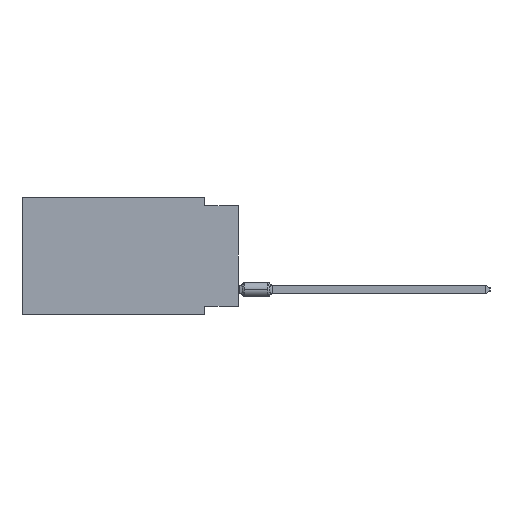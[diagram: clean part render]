
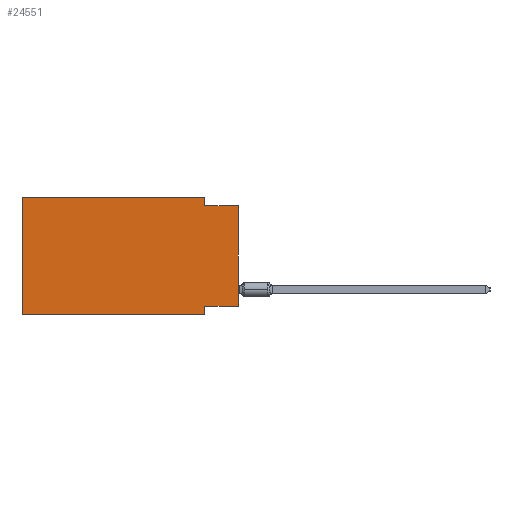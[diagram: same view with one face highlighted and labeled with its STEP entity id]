
A CAD part, left-side view. The second image highlights one B-rep face of the part: STEP entity #24551.
In plain terms, the highlighted planar face has unit normal (-1, 0, 0).
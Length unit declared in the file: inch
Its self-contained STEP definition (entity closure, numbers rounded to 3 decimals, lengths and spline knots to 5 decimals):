
#3722 = CARTESIAN_POINT ( 'NONE',  ( 0., 0.1, -0.35 ) ) ;
#4383 = EDGE_CURVE ( 'NONE', #33869, #52379, #29359, .T. ) ;
#4800 = PLANE ( 'NONE',  #45881 ) ;
#4854 = VECTOR ( 'NONE', #38782, 39.37008 ) ;
#5551 = CARTESIAN_POINT ( 'NONE',  ( 0., 0.645, -0.35 ) ) ;
#7350 = VERTEX_POINT ( 'NONE', #24100 ) ;
#8045 = CARTESIAN_POINT ( 'NONE',  ( 0., 0.645, 0. ) ) ;
#9437 = ORIENTED_EDGE ( 'NONE', *, *, #50084, .F. ) ;
#10578 = ORIENTED_EDGE ( 'NONE', *, *, #64224, .T. ) ;
#11605 = EDGE_CURVE ( 'NONE', #21707, #7350, #18316, .T. ) ;
#14691 = CARTESIAN_POINT ( 'NONE',  ( 0., 0.1, -0.025 ) ) ;
#14820 = DIRECTION ( 'NONE',  ( 0., 0., -1. ) ) ;
#15753 = DIRECTION ( 'NONE',  ( 1., 0., 0. ) ) ;
#16477 = DIRECTION ( 'NONE',  ( 0., 0., -1. ) ) ;
#18316 = LINE ( 'NONE', #50862, #23615 ) ;
#18768 = LINE ( 'NONE', #24285, #55905 ) ;
#21707 = VERTEX_POINT ( 'NONE', #14691 ) ;
#23089 = EDGE_CURVE ( 'NONE', #51325, #28256, #49789, .T. ) ;
#23615 = VECTOR ( 'NONE', #57078, 39.37008 ) ;
#23792 = LINE ( 'NONE', #8045, #57624 ) ;
#23897 = CARTESIAN_POINT ( 'NONE',  ( 0., 0., -0.325 ) ) ;
#24100 = CARTESIAN_POINT ( 'NONE',  ( 0., 0., -0.025 ) ) ;
#24285 = CARTESIAN_POINT ( 'NONE',  ( 0., 0., 0. ) ) ;
#24551 = ADVANCED_FACE ( 'NONE', ( #66188 ), #4800, .F. ) ;
#25277 = EDGE_CURVE ( 'NONE', #49358, #38225, #23792, .T. ) ;
#25859 = EDGE_CURVE ( 'NONE', #51325, #49358, #39706, .T. ) ;
#26925 = ORIENTED_EDGE ( 'NONE', *, *, #23089, .T. ) ;
#27628 = CARTESIAN_POINT ( 'NONE',  ( 0., 0.1, -0.325 ) ) ;
#27705 = EDGE_LOOP ( 'NONE', ( #10578, #60563, #9437, #46955, #69010, #26925, #33981, #51672 ) ) ;
#28210 = CARTESIAN_POINT ( 'NONE',  ( 0., 0.645, 0. ) ) ;
#28256 = VERTEX_POINT ( 'NONE', #3722 ) ;
#29359 = LINE ( 'NONE', #23897, #39160 ) ;
#30461 = DIRECTION ( 'NONE',  ( 0., 0., 1. ) ) ;
#33422 = LINE ( 'NONE', #46208, #59299 ) ;
#33869 = VERTEX_POINT ( 'NONE', #35996 ) ;
#33981 = ORIENTED_EDGE ( 'NONE', *, *, #50355, .F. ) ;
#35996 = CARTESIAN_POINT ( 'NONE',  ( 0., 0., -0.325 ) ) ;
#36176 = DIRECTION ( 'NONE',  ( 0., -1., 0. ) ) ;
#37686 = CARTESIAN_POINT ( 'NONE',  ( 0., 0.645, 0. ) ) ;
#38188 = CARTESIAN_POINT ( 'NONE',  ( 0., 0.1, 0. ) ) ;
#38225 = VERTEX_POINT ( 'NONE', #42690 ) ;
#38782 = DIRECTION ( 'NONE',  ( 0., -1., 0. ) ) ;
#39160 = VECTOR ( 'NONE', #68464, 39.37008 ) ;
#39706 = LINE ( 'NONE', #61989, #66980 ) ;
#40737 = DIRECTION ( 'NONE',  ( 0., 0., -1. ) ) ;
#42690 = CARTESIAN_POINT ( 'NONE',  ( 0., 0.1, 0. ) ) ;
#45881 = AXIS2_PLACEMENT_3D ( 'NONE', #37686, #15753, #16477 ) ;
#46208 = CARTESIAN_POINT ( 'NONE',  ( 0., 0.1, -0.35 ) ) ;
#46955 = ORIENTED_EDGE ( 'NONE', *, *, #25277, .F. ) ;
#47576 = VECTOR ( 'NONE', #14820, 39.37008 ) ;
#49358 = VERTEX_POINT ( 'NONE', #28210 ) ;
#49594 = DIRECTION ( 'NONE',  ( 0., 0., 1. ) ) ;
#49789 = LINE ( 'NONE', #5551, #4854 ) ;
#50084 = EDGE_CURVE ( 'NONE', #38225, #21707, #71105, .T. ) ;
#50355 = EDGE_CURVE ( 'NONE', #52379, #28256, #33422, .T. ) ;
#50862 = CARTESIAN_POINT ( 'NONE',  ( 0., 0., -0.025 ) ) ;
#51325 = VERTEX_POINT ( 'NONE', #65806 ) ;
#51672 = ORIENTED_EDGE ( 'NONE', *, *, #4383, .F. ) ;
#52379 = VERTEX_POINT ( 'NONE', #27628 ) ;
#55905 = VECTOR ( 'NONE', #30461, 39.37008 ) ;
#57078 = DIRECTION ( 'NONE',  ( 0., -1., 0. ) ) ;
#57624 = VECTOR ( 'NONE', #36176, 39.37008 ) ;
#59299 = VECTOR ( 'NONE', #40737, 39.37008 ) ;
#60563 = ORIENTED_EDGE ( 'NONE', *, *, #11605, .F. ) ;
#61989 = CARTESIAN_POINT ( 'NONE',  ( 0., 0.645, 0. ) ) ;
#64224 = EDGE_CURVE ( 'NONE', #33869, #7350, #18768, .T. ) ;
#65806 = CARTESIAN_POINT ( 'NONE',  ( 0., 0.645, -0.35 ) ) ;
#66188 = FACE_OUTER_BOUND ( 'NONE', #27705, .T. ) ;
#66980 = VECTOR ( 'NONE', #49594, 39.37008 ) ;
#68464 = DIRECTION ( 'NONE',  ( 0., 1., 0. ) ) ;
#69010 = ORIENTED_EDGE ( 'NONE', *, *, #25859, .F. ) ;
#71105 = LINE ( 'NONE', #38188, #47576 ) ;
